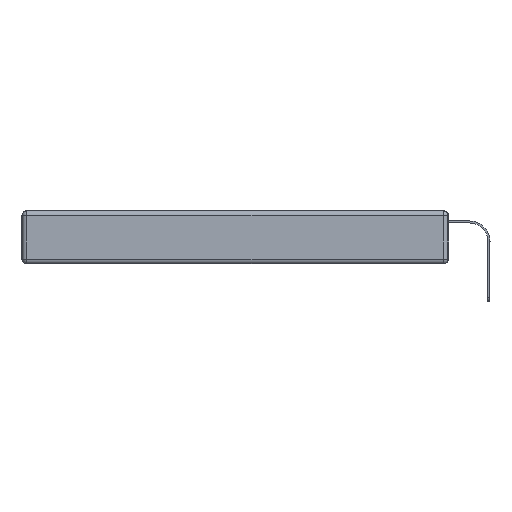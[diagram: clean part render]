
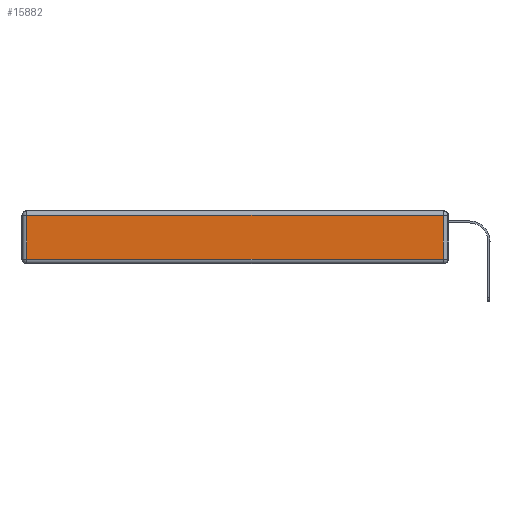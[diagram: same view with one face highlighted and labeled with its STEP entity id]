
A CAD part, left-side view. The second image highlights one B-rep face of the part: STEP entity #15882.
In plain terms, the highlighted planar face has unit normal (-1, 0, 0).
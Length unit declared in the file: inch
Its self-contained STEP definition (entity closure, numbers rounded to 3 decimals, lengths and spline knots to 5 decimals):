
#925 = ORIENTED_EDGE ( 'NONE', *, *, #20388, .T. ) ;
#1037 = CARTESIAN_POINT ( 'NONE',  ( 0., 0.03, -0.313 ) ) ;
#1202 = LINE ( 'NONE', #5108, #14806 ) ;
#1769 = DIRECTION ( 'NONE',  ( 0., 0., 1. ) ) ;
#1879 = PLANE ( 'NONE',  #17441 ) ;
#2156 = CARTESIAN_POINT ( 'NONE',  ( 0., 0., -0.313 ) ) ;
#2210 = EDGE_CURVE ( 'NONE', #3968, #10690, #7144, .T. ) ;
#3762 = VERTEX_POINT ( 'NONE', #21646 ) ;
#3968 = VERTEX_POINT ( 'NONE', #11098 ) ;
#4837 = DIRECTION ( 'NONE',  ( 0., 0., 1. ) ) ;
#5108 = CARTESIAN_POINT ( 'NONE',  ( 0., 2.75, -0.03 ) ) ;
#5931 = DIRECTION ( 'NONE',  ( 0., -1., 0. ) ) ;
#6244 = EDGE_CURVE ( 'NONE', #11228, #3762, #21117, .T. ) ;
#6463 = ORIENTED_EDGE ( 'NONE', *, *, #6244, .T. ) ;
#7144 = LINE ( 'NONE', #21101, #18246 ) ;
#7322 = DIRECTION ( 'NONE',  ( -1., 0., 0. ) ) ;
#9615 = ORIENTED_EDGE ( 'NONE', *, *, #12804, .T. ) ;
#10163 = CARTESIAN_POINT ( 'NONE',  ( 0., 0.03, -0.343 ) ) ;
#10690 = VERTEX_POINT ( 'NONE', #14492 ) ;
#10866 = FACE_OUTER_BOUND ( 'NONE', #16947, .T. ) ;
#11098 = CARTESIAN_POINT ( 'NONE',  ( 0., 2.72, -0.03 ) ) ;
#11228 = VERTEX_POINT ( 'NONE', #1037 ) ;
#12804 = EDGE_CURVE ( 'NONE', #3762, #3968, #1202, .T. ) ;
#14492 = CARTESIAN_POINT ( 'NONE',  ( 0., 2.72, -0.313 ) ) ;
#14806 = VECTOR ( 'NONE', #19592, 39.37008 ) ;
#15882 = ADVANCED_FACE ( 'NONE', ( #10866 ), #1879, .T. ) ;
#16086 = DIRECTION ( 'NONE',  ( 0., 0., -1. ) ) ;
#16947 = EDGE_LOOP ( 'NONE', ( #925, #6463, #9615, #19594 ) ) ;
#17441 = AXIS2_PLACEMENT_3D ( 'NONE', #21927, #7322, #1769 ) ;
#18246 = VECTOR ( 'NONE', #16086, 39.37008 ) ;
#19592 = DIRECTION ( 'NONE',  ( 0., 1., 0. ) ) ;
#19594 = ORIENTED_EDGE ( 'NONE', *, *, #2210, .T. ) ;
#20055 = VECTOR ( 'NONE', #5931, 39.37008 ) ;
#20388 = EDGE_CURVE ( 'NONE', #10690, #11228, #20675, .T. ) ;
#20675 = LINE ( 'NONE', #2156, #20055 ) ;
#21101 = CARTESIAN_POINT ( 'NONE',  ( 0., 2.72, -0.343 ) ) ;
#21117 = LINE ( 'NONE', #10163, #22626 ) ;
#21646 = CARTESIAN_POINT ( 'NONE',  ( 0., 0.03, -0.03 ) ) ;
#21927 = CARTESIAN_POINT ( 'NONE',  ( 0., 0., -0.343 ) ) ;
#22626 = VECTOR ( 'NONE', #4837, 39.37008 ) ;
